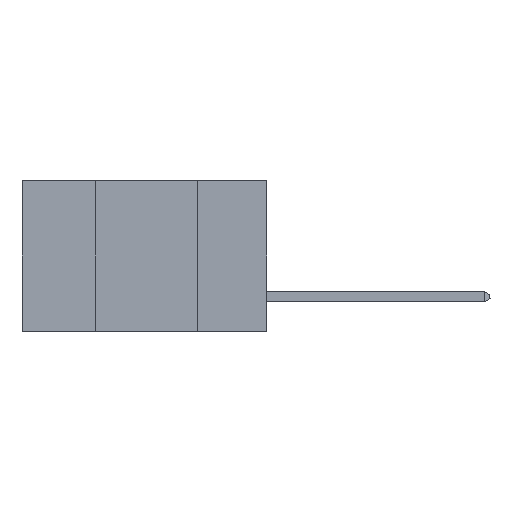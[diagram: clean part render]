
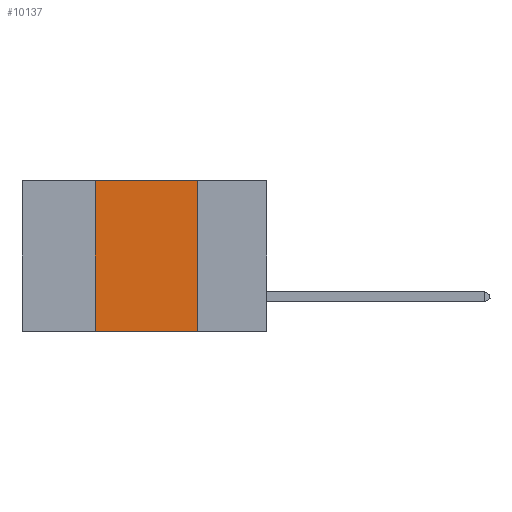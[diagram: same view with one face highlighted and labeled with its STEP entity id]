
A CAD part, left-side view. The second image highlights one B-rep face of the part: STEP entity #10137.
In plain terms, the highlighted planar face has unit normal (-1, 0, 0).
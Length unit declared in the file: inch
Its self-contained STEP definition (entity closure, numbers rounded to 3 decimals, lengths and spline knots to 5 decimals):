
#47 = ORIENTED_EDGE ( 'NONE', *, *, #10416, .F. ) ;
#534 = ORIENTED_EDGE ( 'NONE', *, *, #8458, .F. ) ;
#842 = CARTESIAN_POINT ( 'NONE',  ( 0., 0.6, 0. ) ) ;
#987 = AXIS2_PLACEMENT_3D ( 'NONE', #842, #1791, #7368 ) ;
#1380 = ORIENTED_EDGE ( 'NONE', *, *, #9245, .T. ) ;
#1791 = DIRECTION ( 'NONE',  ( 1., 0., 0. ) ) ;
#1945 = VERTEX_POINT ( 'NONE', #9092 ) ;
#2266 = DIRECTION ( 'NONE',  ( 0., 0., -1. ) ) ;
#2309 = CARTESIAN_POINT ( 'NONE',  ( 0., 0.17, 0. ) ) ;
#2311 = CARTESIAN_POINT ( 'NONE',  ( 0., 0.17, 0. ) ) ;
#2326 = ORIENTED_EDGE ( 'NONE', *, *, #4451, .F. ) ;
#2949 = EDGE_LOOP ( 'NONE', ( #2326, #534, #47, #1380 ) ) ;
#3023 = VERTEX_POINT ( 'NONE', #2309 ) ;
#3674 = CARTESIAN_POINT ( 'NONE',  ( 0., 0.6, -0.37 ) ) ;
#4451 = EDGE_CURVE ( 'NONE', #3023, #1945, #8589, .T. ) ;
#5797 = VERTEX_POINT ( 'NONE', #10556 ) ;
#5922 = VECTOR ( 'NONE', #11893, 39.37008 ) ;
#6335 = PLANE ( 'NONE',  #987 ) ;
#7300 = CARTESIAN_POINT ( 'NONE',  ( 0., 0.6, 0. ) ) ;
#7346 = DIRECTION ( 'NONE',  ( 0., -1., 0. ) ) ;
#7368 = DIRECTION ( 'NONE',  ( 0., 0., -1. ) ) ;
#8084 = LINE ( 'NONE', #3674, #5922 ) ;
#8198 = LINE ( 'NONE', #11670, #8346 ) ;
#8346 = VECTOR ( 'NONE', #9053, 39.37008 ) ;
#8458 = EDGE_CURVE ( 'NONE', #5797, #3023, #8824, .T. ) ;
#8589 = LINE ( 'NONE', #2311, #8718 ) ;
#8718 = VECTOR ( 'NONE', #2266, 39.37008 ) ;
#8779 = FACE_OUTER_BOUND ( 'NONE', #2949, .T. ) ;
#8824 = LINE ( 'NONE', #7300, #10969 ) ;
#9053 = DIRECTION ( 'NONE',  ( 0., 0., 1. ) ) ;
#9092 = CARTESIAN_POINT ( 'NONE',  ( 0., 0.17, -0.37 ) ) ;
#9245 = EDGE_CURVE ( 'NONE', #10132, #1945, #8084, .T. ) ;
#10132 = VERTEX_POINT ( 'NONE', #10175 ) ;
#10137 = ADVANCED_FACE ( 'NONE', ( #8779 ), #6335, .F. ) ;
#10175 = CARTESIAN_POINT ( 'NONE',  ( 0., 0.42, -0.37 ) ) ;
#10416 = EDGE_CURVE ( 'NONE', #10132, #5797, #8198, .T. ) ;
#10556 = CARTESIAN_POINT ( 'NONE',  ( 0., 0.42, 0. ) ) ;
#10969 = VECTOR ( 'NONE', #7346, 39.37008 ) ;
#11670 = CARTESIAN_POINT ( 'NONE',  ( 0., 0.42, 0. ) ) ;
#11893 = DIRECTION ( 'NONE',  ( 0., -1., 0. ) ) ;
